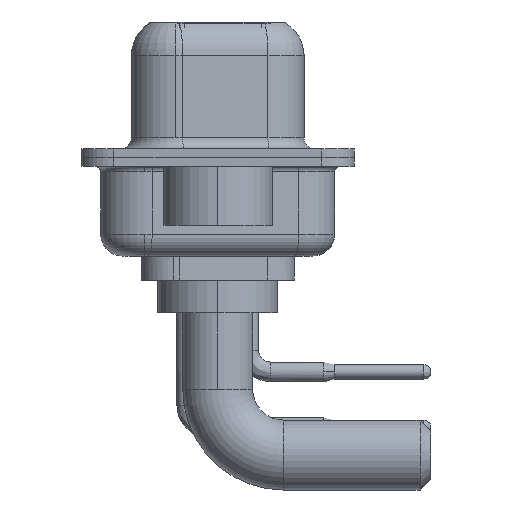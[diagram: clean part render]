
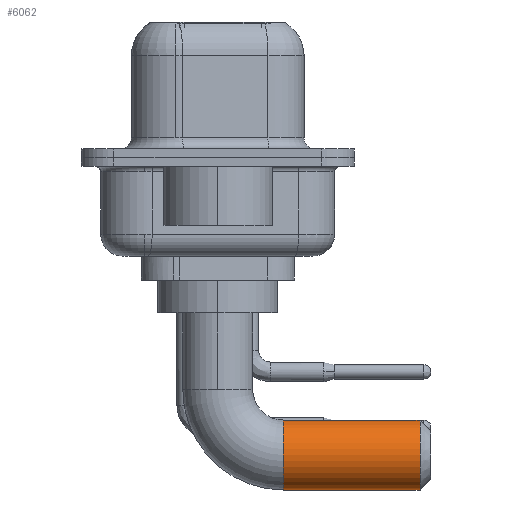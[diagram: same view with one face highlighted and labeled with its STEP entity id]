
A CAD part, left-side view. The second image highlights one B-rep face of the part: STEP entity #6062.
In plain terms, the highlighted cylindrical face has radius 1.6 mm (diameter 3.2 mm), a partial arc.
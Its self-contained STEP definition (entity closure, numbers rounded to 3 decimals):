
#278 = CARTESIAN_POINT ( 'NONE',  ( 0., -3., -4.9 ) ) ;
#750 = VECTOR ( 'NONE', #1428, 1000. ) ;
#943 = DIRECTION ( 'NONE',  ( -1., 0., 0. ) ) ;
#1283 = CYLINDRICAL_SURFACE ( 'NONE', #24082, 1.6 ) ;
#1392 = EDGE_LOOP ( 'NONE', ( #21169, #14196, #12546, #15917 ) ) ;
#1428 = DIRECTION ( 'NONE',  ( 0., -1., 0. ) ) ;
#3058 = DIRECTION ( 'NONE',  ( 0., -1., 0. ) ) ;
#3341 = LINE ( 'NONE', #10750, #750 ) ;
#3712 = VERTEX_POINT ( 'NONE', #23648 ) ;
#3905 = CIRCLE ( 'NONE', #5096, 1.6 ) ;
#4726 = DIRECTION ( 'NONE',  ( 0., -1., 0. ) ) ;
#5096 = AXIS2_PLACEMENT_3D ( 'NONE', #16072, #17485, #6625 ) ;
#5697 = EDGE_CURVE ( 'NONE', #21863, #15805, #3341, .T. ) ;
#6062 = ADVANCED_FACE ( 'NONE', ( #20762 ), #1283, .T. ) ;
#6625 = DIRECTION ( 'NONE',  ( 0., 0., -1. ) ) ;
#7658 = VECTOR ( 'NONE', #9417, 1000. ) ;
#9417 = DIRECTION ( 'NONE',  ( 0., -1., 0. ) ) ;
#10462 = VERTEX_POINT ( 'NONE', #13912 ) ;
#10750 = CARTESIAN_POINT ( 'NONE',  ( 0., -3., -4.9 ) ) ;
#12096 = EDGE_CURVE ( 'NONE', #10462, #3712, #17080, .T. ) ;
#12400 = CARTESIAN_POINT ( 'NONE',  ( 0., -3., -6.5 ) ) ;
#12546 = ORIENTED_EDGE ( 'NONE', *, *, #12096, .T. ) ;
#13912 = CARTESIAN_POINT ( 'NONE',  ( 0., -3., -8.1 ) ) ;
#13951 = AXIS2_PLACEMENT_3D ( 'NONE', #12400, #4726, #943 ) ;
#14196 = ORIENTED_EDGE ( 'NONE', *, *, #18908, .T. ) ;
#15805 = VERTEX_POINT ( 'NONE', #18590 ) ;
#15917 = ORIENTED_EDGE ( 'NONE', *, *, #22301, .T. ) ;
#16072 = CARTESIAN_POINT ( 'NONE',  ( 0., -9.25, -6.5 ) ) ;
#16505 = CARTESIAN_POINT ( 'NONE',  ( 0., -3., -6.5 ) ) ;
#17080 = LINE ( 'NONE', #20969, #7658 ) ;
#17485 = DIRECTION ( 'NONE',  ( 0., 1., 0. ) ) ;
#18590 = CARTESIAN_POINT ( 'NONE',  ( 0., -9.25, -4.9 ) ) ;
#18908 = EDGE_CURVE ( 'NONE', #21863, #10462, #20744, .T. ) ;
#20744 = CIRCLE ( 'NONE', #13951, 1.6 ) ;
#20762 = FACE_OUTER_BOUND ( 'NONE', #1392, .T. ) ;
#20969 = CARTESIAN_POINT ( 'NONE',  ( 0., -3., -8.1 ) ) ;
#21169 = ORIENTED_EDGE ( 'NONE', *, *, #5697, .F. ) ;
#21863 = VERTEX_POINT ( 'NONE', #278 ) ;
#22301 = EDGE_CURVE ( 'NONE', #3712, #15805, #3905, .T. ) ;
#23648 = CARTESIAN_POINT ( 'NONE',  ( 0., -9.25, -8.1 ) ) ;
#24082 = AXIS2_PLACEMENT_3D ( 'NONE', #16505, #3058, #24418 ) ;
#24418 = DIRECTION ( 'NONE',  ( 0., 0., -1. ) ) ;
